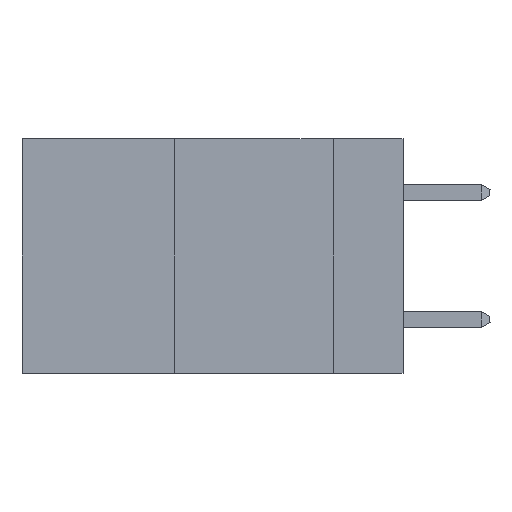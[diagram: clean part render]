
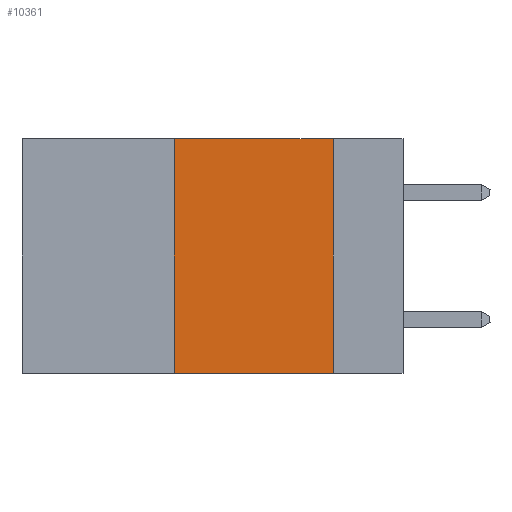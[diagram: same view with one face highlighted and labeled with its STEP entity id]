
A CAD part, left-side view. The second image highlights one B-rep face of the part: STEP entity #10361.
In plain terms, the highlighted planar face has unit normal (-1, 0, 0).
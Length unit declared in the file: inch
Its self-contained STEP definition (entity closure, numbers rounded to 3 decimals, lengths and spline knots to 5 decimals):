
#1171 = AXIS2_PLACEMENT_3D ( 'NONE', #4179, #24405, #9646 ) ;
#2471 = VERTEX_POINT ( 'NONE', #35646 ) ;
#2527 = EDGE_LOOP ( 'NONE', ( #23659, #18636, #21536, #13263 ) ) ;
#4179 = CARTESIAN_POINT ( 'NONE',  ( 0., 0.6, 0. ) ) ;
#4528 = LINE ( 'NONE', #25300, #31812 ) ;
#4600 = VERTEX_POINT ( 'NONE', #4830 ) ;
#4830 = CARTESIAN_POINT ( 'NONE',  ( 0., 0.36, -0.37 ) ) ;
#5817 = LINE ( 'NONE', #25073, #16290 ) ;
#8607 = LINE ( 'NONE', #36691, #27725 ) ;
#8870 = EDGE_CURVE ( 'NONE', #4600, #28993, #8607, .T. ) ;
#9225 = EDGE_CURVE ( 'NONE', #9299, #2471, #20868, .T. ) ;
#9299 = VERTEX_POINT ( 'NONE', #16604 ) ;
#9646 = DIRECTION ( 'NONE',  ( 0., 0., -1. ) ) ;
#10361 = ADVANCED_FACE ( 'NONE', ( #35808 ), #36108, .F. ) ;
#10419 = VECTOR ( 'NONE', #28418, 39.37008 ) ;
#13263 = ORIENTED_EDGE ( 'NONE', *, *, #15290, .T. ) ;
#15290 = EDGE_CURVE ( 'NONE', #4600, #2471, #4528, .T. ) ;
#16290 = VECTOR ( 'NONE', #27975, 39.37008 ) ;
#16604 = CARTESIAN_POINT ( 'NONE',  ( 0., 0.11, 0. ) ) ;
#18636 = ORIENTED_EDGE ( 'NONE', *, *, #30331, .F. ) ;
#19764 = CARTESIAN_POINT ( 'NONE',  ( 0., 0.11, 0. ) ) ;
#20868 = LINE ( 'NONE', #19764, #10419 ) ;
#21536 = ORIENTED_EDGE ( 'NONE', *, *, #8870, .F. ) ;
#22008 = CARTESIAN_POINT ( 'NONE',  ( 0., 0.36, 0. ) ) ;
#22181 = DIRECTION ( 'NONE',  ( 0., 0., 1. ) ) ;
#23659 = ORIENTED_EDGE ( 'NONE', *, *, #9225, .F. ) ;
#24405 = DIRECTION ( 'NONE',  ( 1., 0., 0. ) ) ;
#24654 = DIRECTION ( 'NONE',  ( 0., -1., 0. ) ) ;
#25073 = CARTESIAN_POINT ( 'NONE',  ( 0., 0.6, 0. ) ) ;
#25300 = CARTESIAN_POINT ( 'NONE',  ( 0., 0.6, -0.37 ) ) ;
#27725 = VECTOR ( 'NONE', #22181, 39.37008 ) ;
#27975 = DIRECTION ( 'NONE',  ( 0., -1., 0. ) ) ;
#28418 = DIRECTION ( 'NONE',  ( 0., 0., -1. ) ) ;
#28993 = VERTEX_POINT ( 'NONE', #22008 ) ;
#30331 = EDGE_CURVE ( 'NONE', #28993, #9299, #5817, .T. ) ;
#31812 = VECTOR ( 'NONE', #24654, 39.37008 ) ;
#35646 = CARTESIAN_POINT ( 'NONE',  ( 0., 0.11, -0.37 ) ) ;
#35808 = FACE_OUTER_BOUND ( 'NONE', #2527, .T. ) ;
#36108 = PLANE ( 'NONE',  #1171 ) ;
#36691 = CARTESIAN_POINT ( 'NONE',  ( 0., 0.36, 0. ) ) ;
